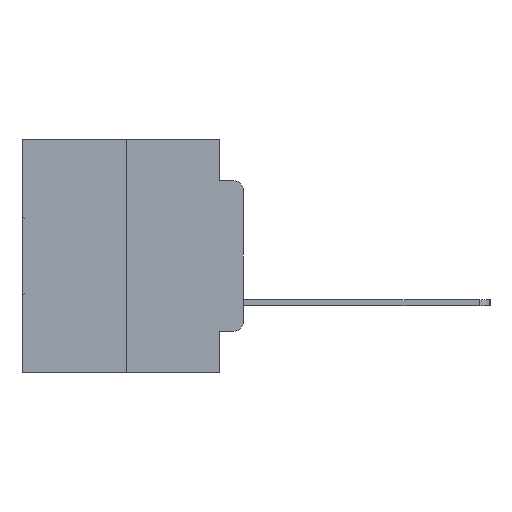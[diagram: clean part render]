
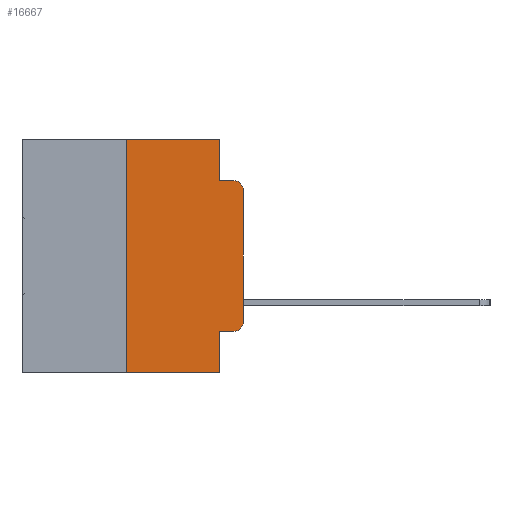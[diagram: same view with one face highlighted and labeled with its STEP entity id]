
A CAD part, left-side view. The second image highlights one B-rep face of the part: STEP entity #16667.
In plain terms, the highlighted planar face has unit normal (-1, 0, 0).
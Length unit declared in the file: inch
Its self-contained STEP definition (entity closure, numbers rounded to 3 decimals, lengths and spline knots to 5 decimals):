
#247 = AXIS2_PLACEMENT_3D ( 'NONE', #10908, #27331, #13339 ) ;
#540 = CARTESIAN_POINT ( 'NONE',  ( 0., 0.051, -0.0885 ) ) ;
#710 = EDGE_CURVE ( 'NONE', #4859, #6905, #26012, .T. ) ;
#1050 = EDGE_CURVE ( 'NONE', #14963, #1250, #10158, .T. ) ;
#1250 = VERTEX_POINT ( 'NONE', #3613 ) ;
#1599 = CARTESIAN_POINT ( 'NONE',  ( 0., 0.051, -0.4115 ) ) ;
#3613 = CARTESIAN_POINT ( 'NONE',  ( 0., 0.02, -0.4115 ) ) ;
#3757 = VECTOR ( 'NONE', #18042, 39.37008 ) ;
#4122 = CARTESIAN_POINT ( 'NONE',  ( 0., 0.25, 0. ) ) ;
#4170 = LINE ( 'NONE', #19654, #28568 ) ;
#4316 = CARTESIAN_POINT ( 'NONE',  ( 0., 0.473, 0. ) ) ;
#4426 = VERTEX_POINT ( 'NONE', #15189 ) ;
#4776 = EDGE_CURVE ( 'NONE', #27477, #28778, #15152, .T. ) ;
#4859 = VERTEX_POINT ( 'NONE', #20135 ) ;
#5006 = EDGE_CURVE ( 'NONE', #14963, #26070, #27222, .T. ) ;
#5039 = EDGE_CURVE ( 'NONE', #30562, #4859, #13328, .T. ) ;
#5043 = LINE ( 'NONE', #20952, #29437 ) ;
#5624 = VECTOR ( 'NONE', #19466, 39.37008 ) ;
#6730 = DIRECTION ( 'NONE',  ( 0., 0., -1. ) ) ;
#6886 = VECTOR ( 'NONE', #27821, 39.37008 ) ;
#6905 = VERTEX_POINT ( 'NONE', #15932 ) ;
#7074 = ORIENTED_EDGE ( 'NONE', *, *, #1050, .T. ) ;
#7774 = EDGE_CURVE ( 'NONE', #13982, #4426, #5043, .T. ) ;
#7793 = ORIENTED_EDGE ( 'NONE', *, *, #10539, .T. ) ;
#7821 = ORIENTED_EDGE ( 'NONE', *, *, #5039, .T. ) ;
#8916 = ORIENTED_EDGE ( 'NONE', *, *, #7774, .F. ) ;
#9788 = LINE ( 'NONE', #17114, #5624 ) ;
#10122 = VECTOR ( 'NONE', #17175, 39.37008 ) ;
#10158 = LINE ( 'NONE', #17024, #3757 ) ;
#10539 = EDGE_CURVE ( 'NONE', #27477, #26070, #9788, .T. ) ;
#10908 = CARTESIAN_POINT ( 'NONE',  ( 0., 0.02, -0.3915 ) ) ;
#11144 = CARTESIAN_POINT ( 'NONE',  ( 0., 0.25, -0.5 ) ) ;
#11157 = EDGE_CURVE ( 'NONE', #4426, #6905, #16403, .T. ) ;
#11619 = DIRECTION ( 'NONE',  ( 0., 0., -1. ) ) ;
#11988 = ORIENTED_EDGE ( 'NONE', *, *, #27856, .F. ) ;
#12600 = CARTESIAN_POINT ( 'NONE',  ( 0., 0., -0.3915 ) ) ;
#13104 = ORIENTED_EDGE ( 'NONE', *, *, #5006, .F. ) ;
#13212 = DIRECTION ( 'NONE',  ( 0., 0., -1. ) ) ;
#13328 = LINE ( 'NONE', #23150, #6886 ) ;
#13339 = DIRECTION ( 'NONE',  ( 0., 0., -1. ) ) ;
#13975 = AXIS2_PLACEMENT_3D ( 'NONE', #24806, #24616, #13212 ) ;
#13982 = VERTEX_POINT ( 'NONE', #23465 ) ;
#14053 = VECTOR ( 'NONE', #27615, 39.37008 ) ;
#14963 = VERTEX_POINT ( 'NONE', #1599 ) ;
#15152 = LINE ( 'NONE', #19730, #20634 ) ;
#15189 = CARTESIAN_POINT ( 'NONE',  ( 0., 0.051, -0.0885 ) ) ;
#15932 = CARTESIAN_POINT ( 'NONE',  ( 0., 0.02, -0.0885 ) ) ;
#15941 = CARTESIAN_POINT ( 'NONE',  ( 0., 0.051, 0. ) ) ;
#16220 = PLANE ( 'NONE',  #29722 ) ;
#16403 = LINE ( 'NONE', #540, #10122 ) ;
#16667 = ADVANCED_FACE ( 'NONE', ( #28205 ), #16220, .F. ) ;
#17024 = CARTESIAN_POINT ( 'NONE',  ( 0., 0.051, -0.4115 ) ) ;
#17114 = CARTESIAN_POINT ( 'NONE',  ( 0., 0.473, -0.5 ) ) ;
#17175 = DIRECTION ( 'NONE',  ( 0., -1., 0. ) ) ;
#18042 = DIRECTION ( 'NONE',  ( 0., -1., 0. ) ) ;
#18660 = CIRCLE ( 'NONE', #247, 0.02 ) ;
#19466 = DIRECTION ( 'NONE',  ( 0., -1., 0. ) ) ;
#19654 = CARTESIAN_POINT ( 'NONE',  ( 0., 0.473, 0. ) ) ;
#19730 = CARTESIAN_POINT ( 'NONE',  ( 0., 0.25, 0. ) ) ;
#20135 = CARTESIAN_POINT ( 'NONE',  ( 0., 0., -0.1085 ) ) ;
#20634 = VECTOR ( 'NONE', #29134, 39.37008 ) ;
#20744 = ORIENTED_EDGE ( 'NONE', *, *, #4776, .F. ) ;
#20929 = DIRECTION ( 'NONE',  ( 1., 0., 0. ) ) ;
#20952 = CARTESIAN_POINT ( 'NONE',  ( 0., 0.051, 0. ) ) ;
#21253 = EDGE_LOOP ( 'NONE', ( #7821, #21523, #26617, #8916, #11988, #20744, #7793, #13104, #7074, #23532 ) ) ;
#21523 = ORIENTED_EDGE ( 'NONE', *, *, #710, .T. ) ;
#23150 = CARTESIAN_POINT ( 'NONE',  ( 0., 0., 0. ) ) ;
#23465 = CARTESIAN_POINT ( 'NONE',  ( 0., 0.051, 0. ) ) ;
#23532 = ORIENTED_EDGE ( 'NONE', *, *, #28002, .T. ) ;
#24616 = DIRECTION ( 'NONE',  ( -1., 0., 0. ) ) ;
#24806 = CARTESIAN_POINT ( 'NONE',  ( 0., 0.02, -0.1085 ) ) ;
#26012 = CIRCLE ( 'NONE', #13975, 0.02 ) ;
#26070 = VERTEX_POINT ( 'NONE', #27444 ) ;
#26617 = ORIENTED_EDGE ( 'NONE', *, *, #11157, .F. ) ;
#26731 = DIRECTION ( 'NONE',  ( 0., -1., 0. ) ) ;
#27222 = LINE ( 'NONE', #15941, #14053 ) ;
#27331 = DIRECTION ( 'NONE',  ( -1., 0., 0. ) ) ;
#27444 = CARTESIAN_POINT ( 'NONE',  ( 0., 0.051, -0.5 ) ) ;
#27477 = VERTEX_POINT ( 'NONE', #11144 ) ;
#27615 = DIRECTION ( 'NONE',  ( 0., 0., -1. ) ) ;
#27821 = DIRECTION ( 'NONE',  ( 0., 0., 1. ) ) ;
#27856 = EDGE_CURVE ( 'NONE', #28778, #13982, #4170, .T. ) ;
#28002 = EDGE_CURVE ( 'NONE', #1250, #30562, #18660, .T. ) ;
#28205 = FACE_OUTER_BOUND ( 'NONE', #21253, .T. ) ;
#28568 = VECTOR ( 'NONE', #26731, 39.37008 ) ;
#28778 = VERTEX_POINT ( 'NONE', #4122 ) ;
#29134 = DIRECTION ( 'NONE',  ( 0., 0., 1. ) ) ;
#29437 = VECTOR ( 'NONE', #11619, 39.37008 ) ;
#29722 = AXIS2_PLACEMENT_3D ( 'NONE', #4316, #20929, #6730 ) ;
#30562 = VERTEX_POINT ( 'NONE', #12600 ) ;
